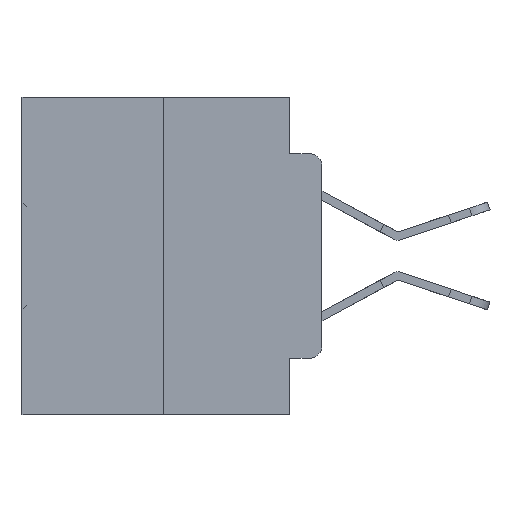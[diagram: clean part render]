
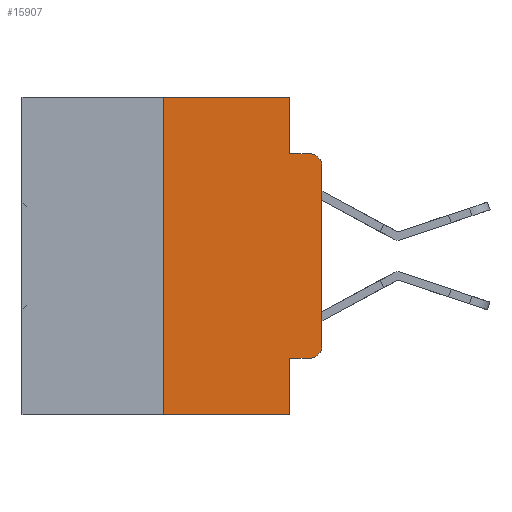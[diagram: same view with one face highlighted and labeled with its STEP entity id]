
A CAD part, left-side view. The second image highlights one B-rep face of the part: STEP entity #15907.
In plain terms, the highlighted planar face has unit normal (-1, 0, 0).
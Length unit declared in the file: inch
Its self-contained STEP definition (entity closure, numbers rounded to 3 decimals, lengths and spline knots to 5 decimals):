
#43 = ORIENTED_EDGE ( 'NONE', *, *, #19268, .F. ) ;
#176 = ORIENTED_EDGE ( 'NONE', *, *, #3158, .F. ) ;
#803 = VECTOR ( 'NONE', #20250, 39.37008 ) ;
#986 = CARTESIAN_POINT ( 'NONE',  ( 0., 0.02, -0.0885 ) ) ;
#1099 = CARTESIAN_POINT ( 'NONE',  ( 0., 0.473, -0.5 ) ) ;
#2210 = CARTESIAN_POINT ( 'NONE',  ( 0., 0.051, 0. ) ) ;
#2664 = DIRECTION ( 'NONE',  ( 0., -1., 0. ) ) ;
#2724 = DIRECTION ( 'NONE',  ( 0., 0., -1. ) ) ;
#2815 = CARTESIAN_POINT ( 'NONE',  ( 0., 0., -0.3915 ) ) ;
#3158 = EDGE_CURVE ( 'NONE', #17428, #33805, #26963, .T. ) ;
#3287 = CARTESIAN_POINT ( 'NONE',  ( 0., 0.473, 0. ) ) ;
#4095 = CARTESIAN_POINT ( 'NONE',  ( 0., 0.02, -0.4115 ) ) ;
#4568 = LINE ( 'NONE', #23251, #5894 ) ;
#5310 = CARTESIAN_POINT ( 'NONE',  ( 0., 0.473, 0. ) ) ;
#5489 = VERTEX_POINT ( 'NONE', #15009 ) ;
#5773 = LINE ( 'NONE', #18607, #13447 ) ;
#5894 = VECTOR ( 'NONE', #6965, 39.37008 ) ;
#6516 = VECTOR ( 'NONE', #2664, 39.37008 ) ;
#6585 = LINE ( 'NONE', #9657, #13000 ) ;
#6685 = CIRCLE ( 'NONE', #23837, 0.02 ) ;
#6743 = ORIENTED_EDGE ( 'NONE', *, *, #25007, .T. ) ;
#6965 = DIRECTION ( 'NONE',  ( 0., -1., 0. ) ) ;
#8298 = LINE ( 'NONE', #26249, #26203 ) ;
#8347 = AXIS2_PLACEMENT_3D ( 'NONE', #3287, #25194, #17003 ) ;
#9616 = ORIENTED_EDGE ( 'NONE', *, *, #13867, .T. ) ;
#9657 = CARTESIAN_POINT ( 'NONE',  ( 0., 0.051, 0. ) ) ;
#10435 = CARTESIAN_POINT ( 'NONE',  ( 0., 0.051, 0. ) ) ;
#10480 = EDGE_CURVE ( 'NONE', #32141, #10826, #5773, .T. ) ;
#10826 = VERTEX_POINT ( 'NONE', #33347 ) ;
#11018 = LINE ( 'NONE', #1099, #31860 ) ;
#11830 = CARTESIAN_POINT ( 'NONE',  ( 0., 0.25, 0. ) ) ;
#12313 = VERTEX_POINT ( 'NONE', #4095 ) ;
#12343 = DIRECTION ( 'NONE',  ( 0., 0., -1. ) ) ;
#12391 = EDGE_CURVE ( 'NONE', #5489, #21790, #4568, .T. ) ;
#13000 = VECTOR ( 'NONE', #25971, 39.37008 ) ;
#13239 = ORIENTED_EDGE ( 'NONE', *, *, #28638, .T. ) ;
#13447 = VECTOR ( 'NONE', #21550, 39.37008 ) ;
#13867 = EDGE_CURVE ( 'NONE', #18435, #12313, #8298, .T. ) ;
#15009 = CARTESIAN_POINT ( 'NONE',  ( 0., 0.051, -0.0885 ) ) ;
#15308 = CARTESIAN_POINT ( 'NONE',  ( 0., 0.02, -0.1085 ) ) ;
#15501 = EDGE_LOOP ( 'NONE', ( #31903, #6743, #21089, #32163, #176, #43, #13239, #16005, #9616, #18977 ) ) ;
#15907 = ADVANCED_FACE ( 'NONE', ( #28145 ), #25299, .F. ) ;
#16005 = ORIENTED_EDGE ( 'NONE', *, *, #16379, .F. ) ;
#16379 = EDGE_CURVE ( 'NONE', #18435, #25780, #25581, .T. ) ;
#16458 = VERTEX_POINT ( 'NONE', #21836 ) ;
#16793 = DIRECTION ( 'NONE',  ( -1., 0., 0. ) ) ;
#17003 = DIRECTION ( 'NONE',  ( 0., 0., -1. ) ) ;
#17428 = VERTEX_POINT ( 'NONE', #11830 ) ;
#18435 = VERTEX_POINT ( 'NONE', #23755 ) ;
#18607 = CARTESIAN_POINT ( 'NONE',  ( 0., 0., 0. ) ) ;
#18947 = CARTESIAN_POINT ( 'NONE',  ( 0., 0.051, -0.5 ) ) ;
#18977 = ORIENTED_EDGE ( 'NONE', *, *, #31636, .T. ) ;
#19268 = EDGE_CURVE ( 'NONE', #16458, #17428, #29783, .T. ) ;
#20250 = DIRECTION ( 'NONE',  ( 0., 0., 1. ) ) ;
#20368 = AXIS2_PLACEMENT_3D ( 'NONE', #29984, #16793, #2724 ) ;
#21089 = ORIENTED_EDGE ( 'NONE', *, *, #12391, .F. ) ;
#21484 = DIRECTION ( 'NONE',  ( 0., 0., -1. ) ) ;
#21550 = DIRECTION ( 'NONE',  ( 0., 0., 1. ) ) ;
#21790 = VERTEX_POINT ( 'NONE', #986 ) ;
#21836 = CARTESIAN_POINT ( 'NONE',  ( 0., 0.25, -0.5 ) ) ;
#22999 = DIRECTION ( 'NONE',  ( 0., -1., 0. ) ) ;
#23251 = CARTESIAN_POINT ( 'NONE',  ( 0., 0.051, -0.0885 ) ) ;
#23755 = CARTESIAN_POINT ( 'NONE',  ( 0., 0.051, -0.4115 ) ) ;
#23837 = AXIS2_PLACEMENT_3D ( 'NONE', #15308, #28589, #12343 ) ;
#25007 = EDGE_CURVE ( 'NONE', #10826, #21790, #6685, .T. ) ;
#25194 = DIRECTION ( 'NONE',  ( 1., 0., 0. ) ) ;
#25299 = PLANE ( 'NONE',  #8347 ) ;
#25581 = LINE ( 'NONE', #10435, #33654 ) ;
#25780 = VERTEX_POINT ( 'NONE', #18947 ) ;
#25971 = DIRECTION ( 'NONE',  ( 0., 0., -1. ) ) ;
#26203 = VECTOR ( 'NONE', #29327, 39.37008 ) ;
#26249 = CARTESIAN_POINT ( 'NONE',  ( 0., 0.051, -0.4115 ) ) ;
#26963 = LINE ( 'NONE', #5310, #6516 ) ;
#28145 = FACE_OUTER_BOUND ( 'NONE', #15501, .T. ) ;
#28589 = DIRECTION ( 'NONE',  ( -1., 0., 0. ) ) ;
#28638 = EDGE_CURVE ( 'NONE', #16458, #25780, #11018, .T. ) ;
#29327 = DIRECTION ( 'NONE',  ( 0., -1., 0. ) ) ;
#29783 = LINE ( 'NONE', #33790, #803 ) ;
#29984 = CARTESIAN_POINT ( 'NONE',  ( 0., 0.02, -0.3915 ) ) ;
#31175 = EDGE_CURVE ( 'NONE', #33805, #5489, #6585, .T. ) ;
#31636 = EDGE_CURVE ( 'NONE', #12313, #32141, #31683, .T. ) ;
#31683 = CIRCLE ( 'NONE', #20368, 0.02 ) ;
#31860 = VECTOR ( 'NONE', #22999, 39.37008 ) ;
#31903 = ORIENTED_EDGE ( 'NONE', *, *, #10480, .T. ) ;
#32141 = VERTEX_POINT ( 'NONE', #2815 ) ;
#32163 = ORIENTED_EDGE ( 'NONE', *, *, #31175, .F. ) ;
#33347 = CARTESIAN_POINT ( 'NONE',  ( 0., 0., -0.1085 ) ) ;
#33654 = VECTOR ( 'NONE', #21484, 39.37008 ) ;
#33790 = CARTESIAN_POINT ( 'NONE',  ( 0., 0.25, 0. ) ) ;
#33805 = VERTEX_POINT ( 'NONE', #2210 ) ;
